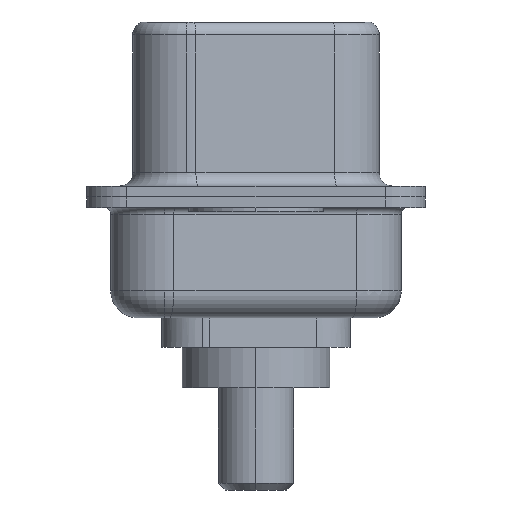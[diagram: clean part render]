
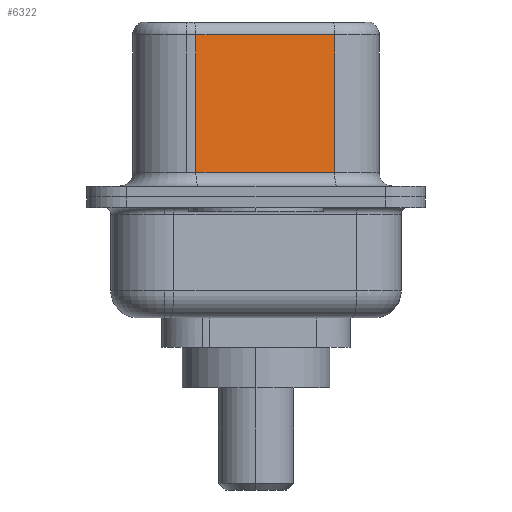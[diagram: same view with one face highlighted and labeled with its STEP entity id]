
A CAD part, left-side view. The second image highlights one B-rep face of the part: STEP entity #6322.
In plain terms, the highlighted planar face has unit normal (-0.985, -0.174, 0).
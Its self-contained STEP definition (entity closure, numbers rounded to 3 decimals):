
#8 = VECTOR ( 'NONE', #1197, 1000. ) ;
#116 = CARTESIAN_POINT ( 'NONE',  ( 4.58, -2.927, 6.52 ) ) ;
#828 = DIRECTION ( 'NONE',  ( -0.174, 0.985, 0. ) ) ;
#984 = VERTEX_POINT ( 'NONE', #6118 ) ;
#1195 = EDGE_LOOP ( 'NONE', ( #9491, #4853, #10276, #2865 ) ) ;
#1197 = DIRECTION ( 'NONE',  ( 0.174, -0.985, 0. ) ) ;
#1405 = EDGE_CURVE ( 'NONE', #984, #8082, #2727, .T. ) ;
#1548 = CARTESIAN_POINT ( 'NONE',  ( 4.58, -2.927, 0.9 ) ) ;
#1571 = PLANE ( 'NONE',  #7949 ) ;
#1700 = LINE ( 'NONE', #116, #4030 ) ;
#1859 = CARTESIAN_POINT ( 'NONE',  ( 4.58, -2.927, 6.02 ) ) ;
#2200 = VERTEX_POINT ( 'NONE', #9281 ) ;
#2300 = CARTESIAN_POINT ( 'NONE',  ( 4.58, -2.927, 6.02 ) ) ;
#2727 = LINE ( 'NONE', #9197, #8 ) ;
#2865 = ORIENTED_EDGE ( 'NONE', *, *, #1405, .T. ) ;
#4030 = VECTOR ( 'NONE', #11560, 1000. ) ;
#4853 = ORIENTED_EDGE ( 'NONE', *, *, #10298, .T. ) ;
#6118 = CARTESIAN_POINT ( 'NONE',  ( 3.67, 2.233, 0.9 ) ) ;
#6322 = ADVANCED_FACE ( 'NONE', ( #10529 ), #1571, .F. ) ;
#6947 = VECTOR ( 'NONE', #12079, 1000. ) ;
#7506 = CARTESIAN_POINT ( 'NONE',  ( 3.67, 2.233, 6.52 ) ) ;
#7949 = AXIS2_PLACEMENT_3D ( 'NONE', #11246, #10816, #8194 ) ;
#8082 = VERTEX_POINT ( 'NONE', #1548 ) ;
#8194 = DIRECTION ( 'NONE',  ( -0.174, 0.985, 0. ) ) ;
#8347 = EDGE_CURVE ( 'NONE', #11374, #8082, #1700, .T. ) ;
#9197 = CARTESIAN_POINT ( 'NONE',  ( 4.58, -2.927, 0.9 ) ) ;
#9281 = CARTESIAN_POINT ( 'NONE',  ( 3.67, 2.233, 6.02 ) ) ;
#9491 = ORIENTED_EDGE ( 'NONE', *, *, #8347, .F. ) ;
#9730 = EDGE_CURVE ( 'NONE', #2200, #984, #11303, .T. ) ;
#9845 = LINE ( 'NONE', #1859, #12028 ) ;
#10276 = ORIENTED_EDGE ( 'NONE', *, *, #9730, .T. ) ;
#10298 = EDGE_CURVE ( 'NONE', #11374, #2200, #9845, .T. ) ;
#10529 = FACE_OUTER_BOUND ( 'NONE', #1195, .T. ) ;
#10816 = DIRECTION ( 'NONE',  ( 0.985, 0.174, 0. ) ) ;
#11246 = CARTESIAN_POINT ( 'NONE',  ( 4.58, -2.927, 6.52 ) ) ;
#11303 = LINE ( 'NONE', #7506, #6947 ) ;
#11374 = VERTEX_POINT ( 'NONE', #2300 ) ;
#11560 = DIRECTION ( 'NONE',  ( 0., 0., -1. ) ) ;
#12028 = VECTOR ( 'NONE', #828, 1000. ) ;
#12079 = DIRECTION ( 'NONE',  ( 0., 0., -1. ) ) ;
